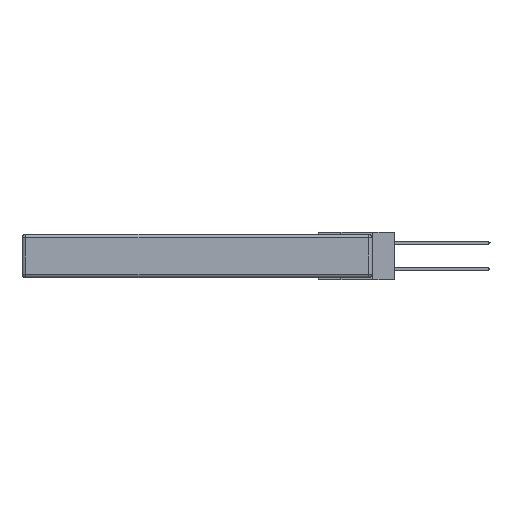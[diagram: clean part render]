
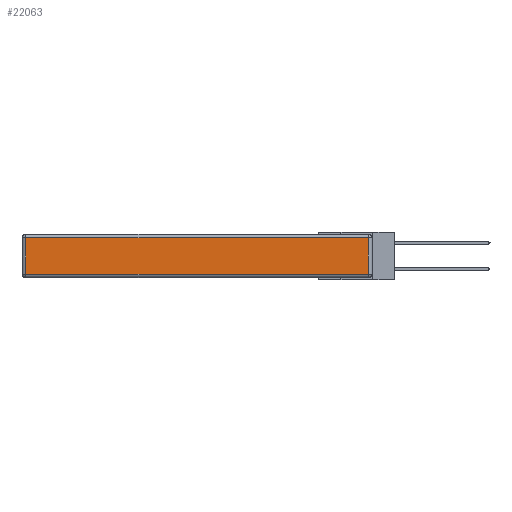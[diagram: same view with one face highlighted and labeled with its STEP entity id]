
A CAD part, left-side view. The second image highlights one B-rep face of the part: STEP entity #22063.
In plain terms, the highlighted planar face has unit normal (-1, 0, 0).
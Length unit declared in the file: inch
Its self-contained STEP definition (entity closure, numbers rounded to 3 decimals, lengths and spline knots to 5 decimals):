
#112 = ORIENTED_EDGE ( 'NONE', *, *, #5504, .T. ) ;
#1615 = LINE ( 'NONE', #5417, #24491 ) ;
#2553 = CARTESIAN_POINT ( 'NONE',  ( 0., 0.03, -0.03 ) ) ;
#2903 = VERTEX_POINT ( 'NONE', #22321 ) ;
#3248 = LINE ( 'NONE', #10948, #23616 ) ;
#5150 = VERTEX_POINT ( 'NONE', #9899 ) ;
#5182 = DIRECTION ( 'NONE',  ( 0., 1., 0. ) ) ;
#5417 = CARTESIAN_POINT ( 'NONE',  ( 0., 0., -0.313 ) ) ;
#5473 = AXIS2_PLACEMENT_3D ( 'NONE', #16550, #10394, #10655 ) ;
#5504 = EDGE_CURVE ( 'NONE', #17587, #17281, #17435, .T. ) ;
#5678 = EDGE_CURVE ( 'NONE', #2903, #17587, #3248, .T. ) ;
#6165 = CARTESIAN_POINT ( 'NONE',  ( 0., 2.72, -0.03 ) ) ;
#6750 = ORIENTED_EDGE ( 'NONE', *, *, #5678, .T. ) ;
#7033 = CARTESIAN_POINT ( 'NONE',  ( 0., 2.72, -0.343 ) ) ;
#7179 = VECTOR ( 'NONE', #5182, 39.37008 ) ;
#8918 = ORIENTED_EDGE ( 'NONE', *, *, #21035, .T. ) ;
#9899 = CARTESIAN_POINT ( 'NONE',  ( 0., 2.72, -0.313 ) ) ;
#10394 = DIRECTION ( 'NONE',  ( -1., 0., 0. ) ) ;
#10655 = DIRECTION ( 'NONE',  ( 0., 0., 1. ) ) ;
#10948 = CARTESIAN_POINT ( 'NONE',  ( 0., 0.03, -0.343 ) ) ;
#10955 = VECTOR ( 'NONE', #11231, 39.37008 ) ;
#11231 = DIRECTION ( 'NONE',  ( 0., 0., -1. ) ) ;
#12774 = DIRECTION ( 'NONE',  ( 0., 0., 1. ) ) ;
#13391 = DIRECTION ( 'NONE',  ( 0., -1., 0. ) ) ;
#14389 = EDGE_LOOP ( 'NONE', ( #22914, #6750, #112, #8918 ) ) ;
#16550 = CARTESIAN_POINT ( 'NONE',  ( 0., 0., -0.343 ) ) ;
#16856 = LINE ( 'NONE', #7033, #10955 ) ;
#17281 = VERTEX_POINT ( 'NONE', #6165 ) ;
#17435 = LINE ( 'NONE', #23157, #7179 ) ;
#17587 = VERTEX_POINT ( 'NONE', #2553 ) ;
#18474 = PLANE ( 'NONE',  #5473 ) ;
#18948 = EDGE_CURVE ( 'NONE', #5150, #2903, #1615, .T. ) ;
#21035 = EDGE_CURVE ( 'NONE', #17281, #5150, #16856, .T. ) ;
#22063 = ADVANCED_FACE ( 'NONE', ( #22959 ), #18474, .T. ) ;
#22321 = CARTESIAN_POINT ( 'NONE',  ( 0., 0.03, -0.313 ) ) ;
#22914 = ORIENTED_EDGE ( 'NONE', *, *, #18948, .T. ) ;
#22959 = FACE_OUTER_BOUND ( 'NONE', #14389, .T. ) ;
#23157 = CARTESIAN_POINT ( 'NONE',  ( 0., 2.75, -0.03 ) ) ;
#23616 = VECTOR ( 'NONE', #12774, 39.37008 ) ;
#24491 = VECTOR ( 'NONE', #13391, 39.37008 ) ;
